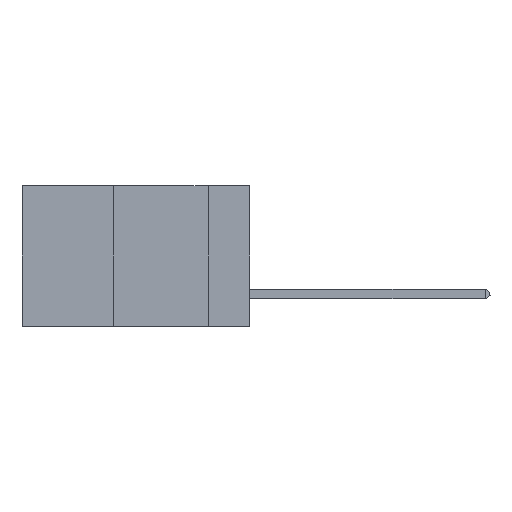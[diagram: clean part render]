
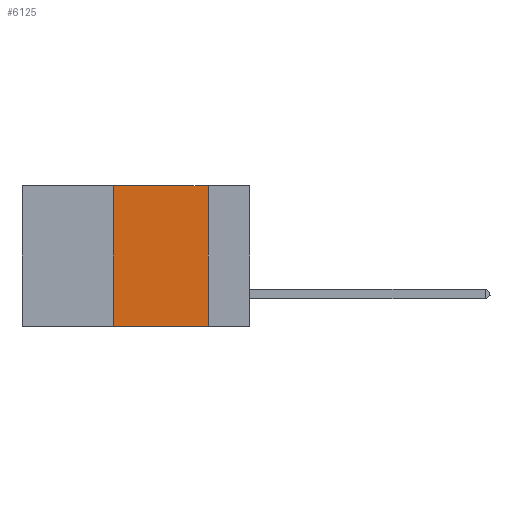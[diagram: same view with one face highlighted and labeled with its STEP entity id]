
A CAD part, left-side view. The second image highlights one B-rep face of the part: STEP entity #6125.
In plain terms, the highlighted planar face has unit normal (-1, 0, 0).
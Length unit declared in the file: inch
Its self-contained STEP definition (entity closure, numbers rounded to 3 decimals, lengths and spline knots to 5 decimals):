
#41 = LINE ( 'NONE', #21045, #18648 ) ;
#628 = CARTESIAN_POINT ( 'NONE',  ( 0., 0.11, 0. ) ) ;
#2069 = VERTEX_POINT ( 'NONE', #3483 ) ;
#2365 = CARTESIAN_POINT ( 'NONE',  ( 0., 0.6, -0.37 ) ) ;
#2370 = DIRECTION ( 'NONE',  ( 0., 0., -1. ) ) ;
#3061 = AXIS2_PLACEMENT_3D ( 'NONE', #3806, #7403, #10998 ) ;
#3082 = EDGE_CURVE ( 'NONE', #9866, #16525, #14433, .T. ) ;
#3362 = VERTEX_POINT ( 'NONE', #13524 ) ;
#3483 = CARTESIAN_POINT ( 'NONE',  ( 0., 0.36, 0. ) ) ;
#3806 = CARTESIAN_POINT ( 'NONE',  ( 0., 0.6, 0. ) ) ;
#3871 = EDGE_CURVE ( 'NONE', #3362, #2069, #41, .T. ) ;
#4418 = ORIENTED_EDGE ( 'NONE', *, *, #3082, .F. ) ;
#4919 = ORIENTED_EDGE ( 'NONE', *, *, #11492, .F. ) ;
#5852 = LINE ( 'NONE', #2365, #20524 ) ;
#6125 = ADVANCED_FACE ( 'NONE', ( #19933 ), #7627, .F. ) ;
#6210 = VECTOR ( 'NONE', #8035, 39.37008 ) ;
#7403 = DIRECTION ( 'NONE',  ( 1., 0., 0. ) ) ;
#7627 = PLANE ( 'NONE',  #3061 ) ;
#8022 = ORIENTED_EDGE ( 'NONE', *, *, #14331, .T. ) ;
#8035 = DIRECTION ( 'NONE',  ( 0., -1., 0. ) ) ;
#8182 = EDGE_LOOP ( 'NONE', ( #4418, #4919, #18548, #8022 ) ) ;
#8372 = LINE ( 'NONE', #19043, #6210 ) ;
#9866 = VERTEX_POINT ( 'NONE', #12800 ) ;
#10998 = DIRECTION ( 'NONE',  ( 0., 0., -1. ) ) ;
#11492 = EDGE_CURVE ( 'NONE', #2069, #9866, #8372, .T. ) ;
#12800 = CARTESIAN_POINT ( 'NONE',  ( 0., 0.11, 0. ) ) ;
#12911 = DIRECTION ( 'NONE',  ( 0., -1., 0. ) ) ;
#13524 = CARTESIAN_POINT ( 'NONE',  ( 0., 0.36, -0.37 ) ) ;
#14200 = VECTOR ( 'NONE', #2370, 39.37008 ) ;
#14331 = EDGE_CURVE ( 'NONE', #3362, #16525, #5852, .T. ) ;
#14433 = LINE ( 'NONE', #628, #14200 ) ;
#16525 = VERTEX_POINT ( 'NONE', #20891 ) ;
#18548 = ORIENTED_EDGE ( 'NONE', *, *, #3871, .F. ) ;
#18648 = VECTOR ( 'NONE', #21159, 39.37008 ) ;
#19043 = CARTESIAN_POINT ( 'NONE',  ( 0., 0.6, 0. ) ) ;
#19933 = FACE_OUTER_BOUND ( 'NONE', #8182, .T. ) ;
#20524 = VECTOR ( 'NONE', #12911, 39.37008 ) ;
#20891 = CARTESIAN_POINT ( 'NONE',  ( 0., 0.11, -0.37 ) ) ;
#21045 = CARTESIAN_POINT ( 'NONE',  ( 0., 0.36, 0. ) ) ;
#21159 = DIRECTION ( 'NONE',  ( 0., 0., 1. ) ) ;
